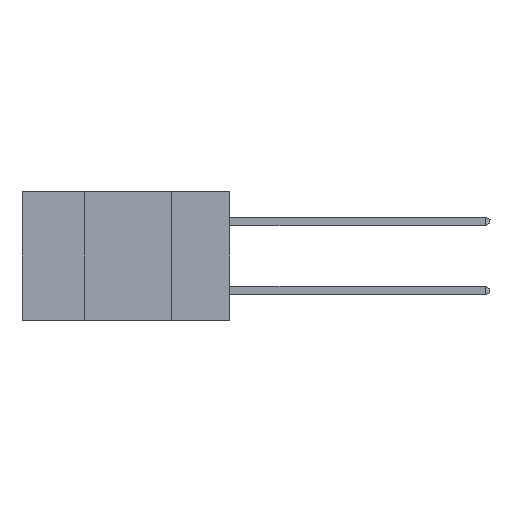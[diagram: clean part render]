
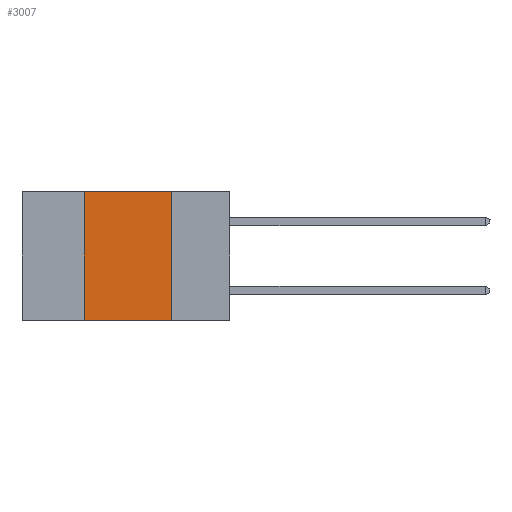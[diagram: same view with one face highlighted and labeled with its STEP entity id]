
A CAD part, left-side view. The second image highlights one B-rep face of the part: STEP entity #3007.
In plain terms, the highlighted planar face has unit normal (-1, 0, 0).
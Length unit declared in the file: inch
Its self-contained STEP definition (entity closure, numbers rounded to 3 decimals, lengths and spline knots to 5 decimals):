
#993 = CARTESIAN_POINT ( 'NONE',  ( 0., 0.42, 0. ) ) ;
#1391 = ORIENTED_EDGE ( 'NONE', *, *, #2423, .F. ) ;
#1643 = LINE ( 'NONE', #13183, #16206 ) ;
#2423 = EDGE_CURVE ( 'NONE', #4801, #18793, #3079, .T. ) ;
#2881 = EDGE_LOOP ( 'NONE', ( #1391, #15447, #9999, #4528 ) ) ;
#3007 = ADVANCED_FACE ( 'NONE', ( #7937 ), #4526, .F. ) ;
#3079 = LINE ( 'NONE', #4354, #14838 ) ;
#4173 = DIRECTION ( 'NONE',  ( 0., -1., 0. ) ) ;
#4354 = CARTESIAN_POINT ( 'NONE',  ( 0., 0.17, -0.37 ) ) ;
#4526 = PLANE ( 'NONE',  #16410 ) ;
#4528 = ORIENTED_EDGE ( 'NONE', *, *, #14177, .T. ) ;
#4801 = VERTEX_POINT ( 'NONE', #6461 ) ;
#6461 = CARTESIAN_POINT ( 'NONE',  ( 0., 0.17, 0. ) ) ;
#6518 = LINE ( 'NONE', #16876, #7808 ) ;
#6519 = EDGE_CURVE ( 'NONE', #17526, #12191, #18173, .T. ) ;
#7808 = VECTOR ( 'NONE', #18738, 39.37008 ) ;
#7937 = FACE_OUTER_BOUND ( 'NONE', #2881, .T. ) ;
#8027 = DIRECTION ( 'NONE',  ( 1., 0., 0. ) ) ;
#8104 = DIRECTION ( 'NONE',  ( 0., 0., 1. ) ) ;
#8388 = EDGE_CURVE ( 'NONE', #12191, #4801, #6518, .T. ) ;
#8702 = VECTOR ( 'NONE', #8104, 39.37008 ) ;
#9501 = CARTESIAN_POINT ( 'NONE',  ( 0., 0.6, 0. ) ) ;
#9999 = ORIENTED_EDGE ( 'NONE', *, *, #6519, .F. ) ;
#10771 = CARTESIAN_POINT ( 'NONE',  ( 0., 0.42, -0.37 ) ) ;
#11369 = CARTESIAN_POINT ( 'NONE',  ( 0., 0.42, -0.37 ) ) ;
#12191 = VERTEX_POINT ( 'NONE', #993 ) ;
#13183 = CARTESIAN_POINT ( 'NONE',  ( 0., 0.6, -0.37 ) ) ;
#14177 = EDGE_CURVE ( 'NONE', #17526, #18793, #1643, .T. ) ;
#14838 = VECTOR ( 'NONE', #17956, 39.37008 ) ;
#15447 = ORIENTED_EDGE ( 'NONE', *, *, #8388, .F. ) ;
#16206 = VECTOR ( 'NONE', #4173, 39.37008 ) ;
#16410 = AXIS2_PLACEMENT_3D ( 'NONE', #9501, #8027, #16452 ) ;
#16452 = DIRECTION ( 'NONE',  ( 0., 0., -1. ) ) ;
#16876 = CARTESIAN_POINT ( 'NONE',  ( 0., 0.6, 0. ) ) ;
#17526 = VERTEX_POINT ( 'NONE', #11369 ) ;
#17956 = DIRECTION ( 'NONE',  ( 0., 0., -1. ) ) ;
#18173 = LINE ( 'NONE', #10771, #8702 ) ;
#18220 = CARTESIAN_POINT ( 'NONE',  ( 0., 0.17, -0.37 ) ) ;
#18738 = DIRECTION ( 'NONE',  ( 0., -1., 0. ) ) ;
#18793 = VERTEX_POINT ( 'NONE', #18220 ) ;
